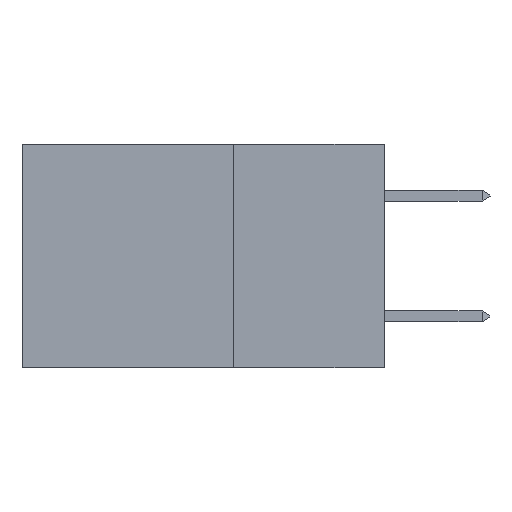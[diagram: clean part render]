
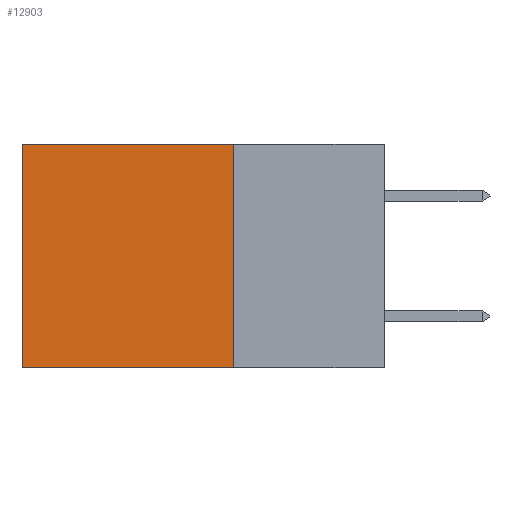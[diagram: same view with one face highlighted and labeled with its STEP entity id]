
A CAD part, left-side view. The second image highlights one B-rep face of the part: STEP entity #12903.
In plain terms, the highlighted planar face has unit normal (-1, 0, 0).
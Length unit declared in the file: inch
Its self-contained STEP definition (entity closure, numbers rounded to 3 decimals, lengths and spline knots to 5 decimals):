
#32 = AXIS2_PLACEMENT_3D ( 'NONE', #4123, #13616, #1707 ) ;
#277 = CARTESIAN_POINT ( 'NONE',  ( 0.2875, 0.25, -0.37 ) ) ;
#289 = EDGE_CURVE ( 'NONE', #4626, #4807, #13683, .T. ) ;
#645 = CARTESIAN_POINT ( 'NONE',  ( 0.2875, 0.6, 0. ) ) ;
#1707 = DIRECTION ( 'NONE',  ( 0., 0., -1. ) ) ;
#1817 = DIRECTION ( 'NONE',  ( 0., 1., 0. ) ) ;
#2262 = EDGE_CURVE ( 'NONE', #11503, #4807, #4722, .T. ) ;
#2771 = ORIENTED_EDGE ( 'NONE', *, *, #3128, .T. ) ;
#3128 = EDGE_CURVE ( 'NONE', #12269, #4626, #6218, .T. ) ;
#3304 = CARTESIAN_POINT ( 'NONE',  ( 0.2875, 0.6, 0. ) ) ;
#3594 = DIRECTION ( 'NONE',  ( 0., 1., 0. ) ) ;
#4123 = CARTESIAN_POINT ( 'NONE',  ( 0.2875, 0.25, 0. ) ) ;
#4150 = ORIENTED_EDGE ( 'NONE', *, *, #9091, .F. ) ;
#4472 = EDGE_LOOP ( 'NONE', ( #4587, #11340, #4150, #2771 ) ) ;
#4587 = ORIENTED_EDGE ( 'NONE', *, *, #289, .T. ) ;
#4626 = VERTEX_POINT ( 'NONE', #3304 ) ;
#4722 = LINE ( 'NONE', #277, #11829 ) ;
#4807 = VERTEX_POINT ( 'NONE', #6131 ) ;
#5042 = FACE_OUTER_BOUND ( 'NONE', #4472, .T. ) ;
#5237 = VECTOR ( 'NONE', #1817, 39.37008 ) ;
#6131 = CARTESIAN_POINT ( 'NONE',  ( 0.2875, 0.6, -0.37 ) ) ;
#6218 = LINE ( 'NONE', #11515, #5237 ) ;
#6240 = DIRECTION ( 'NONE',  ( 0., 0., -1. ) ) ;
#6745 = LINE ( 'NONE', #9963, #12896 ) ;
#8175 = CARTESIAN_POINT ( 'NONE',  ( 0.2875, 0.25, 0. ) ) ;
#9091 = EDGE_CURVE ( 'NONE', #12269, #11503, #6745, .T. ) ;
#9963 = CARTESIAN_POINT ( 'NONE',  ( 0.2875, 0.25, 0. ) ) ;
#10495 = CARTESIAN_POINT ( 'NONE',  ( 0.2875, 0.25, -0.37 ) ) ;
#10955 = DIRECTION ( 'NONE',  ( 0., 0., -1. ) ) ;
#11340 = ORIENTED_EDGE ( 'NONE', *, *, #2262, .F. ) ;
#11503 = VERTEX_POINT ( 'NONE', #10495 ) ;
#11515 = CARTESIAN_POINT ( 'NONE',  ( 0.2875, 0.25, 0. ) ) ;
#11829 = VECTOR ( 'NONE', #3594, 39.37008 ) ;
#11983 = VECTOR ( 'NONE', #6240, 39.37008 ) ;
#12269 = VERTEX_POINT ( 'NONE', #8175 ) ;
#12896 = VECTOR ( 'NONE', #10955, 39.37008 ) ;
#12903 = ADVANCED_FACE ( 'NONE', ( #5042 ), #13538, .F. ) ;
#13538 = PLANE ( 'NONE',  #32 ) ;
#13616 = DIRECTION ( 'NONE',  ( 1., 0., 0. ) ) ;
#13683 = LINE ( 'NONE', #645, #11983 ) ;
